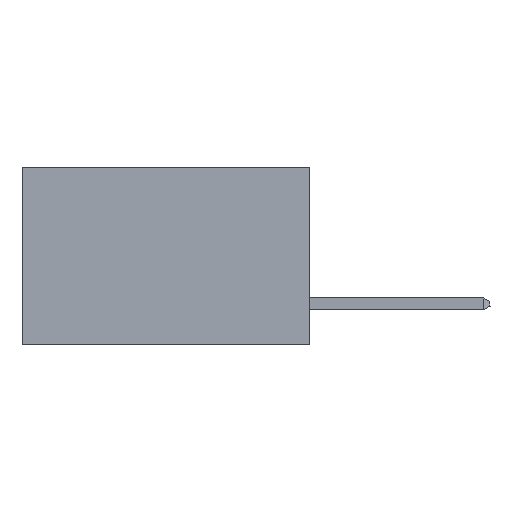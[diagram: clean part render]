
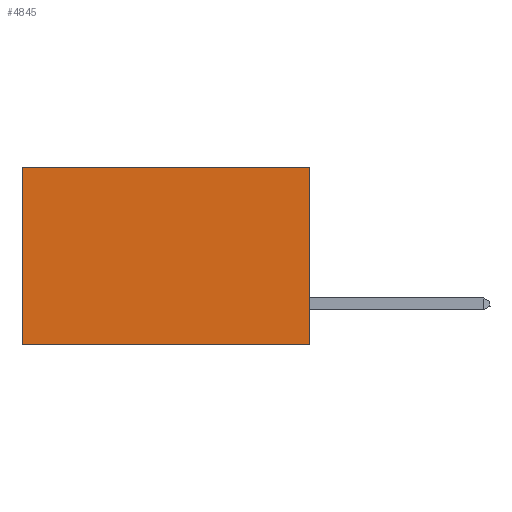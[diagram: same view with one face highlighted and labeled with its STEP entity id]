
A CAD part, left-side view. The second image highlights one B-rep face of the part: STEP entity #4845.
In plain terms, the highlighted planar face has unit normal (-1, 0, 0).
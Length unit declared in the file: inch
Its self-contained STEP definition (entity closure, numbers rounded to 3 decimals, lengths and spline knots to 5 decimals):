
#11 = DIRECTION ( 'NONE',  ( 1., 0., 0. ) ) ;
#539 = DIRECTION ( 'NONE',  ( 0., 0., -1. ) ) ;
#1568 = EDGE_CURVE ( 'NONE', #9355, #11065, #21400, .T. ) ;
#2345 = VECTOR ( 'NONE', #539, 39.37008 ) ;
#4845 = ADVANCED_FACE ( 'NONE', ( #22166 ), #24320, .F. ) ;
#6157 = CARTESIAN_POINT ( 'NONE',  ( 0.2875, 0., 0. ) ) ;
#6753 = VECTOR ( 'NONE', #21107, 39.37008 ) ;
#7283 = CARTESIAN_POINT ( 'NONE',  ( 0.2875, 0.6, -0.37 ) ) ;
#7383 = DIRECTION ( 'NONE',  ( 0., 1., 0. ) ) ;
#7842 = LINE ( 'NONE', #13185, #17094 ) ;
#9315 = CARTESIAN_POINT ( 'NONE',  ( 0.2875, 0.6, 0. ) ) ;
#9355 = VERTEX_POINT ( 'NONE', #9315 ) ;
#10153 = ORIENTED_EDGE ( 'NONE', *, *, #1568, .T. ) ;
#11065 = VERTEX_POINT ( 'NONE', #7283 ) ;
#11925 = CARTESIAN_POINT ( 'NONE',  ( 0.2875, 0., -0.37 ) ) ;
#12388 = VERTEX_POINT ( 'NONE', #22197 ) ;
#13166 = LINE ( 'NONE', #17033, #2345 ) ;
#13185 = CARTESIAN_POINT ( 'NONE',  ( 0.2875, 0., 0. ) ) ;
#14162 = DIRECTION ( 'NONE',  ( 0., 0., -1. ) ) ;
#14805 = EDGE_CURVE ( 'NONE', #12388, #19370, #13166, .T. ) ;
#14972 = CARTESIAN_POINT ( 'NONE',  ( 0.2875, 0.6, 0. ) ) ;
#15254 = EDGE_CURVE ( 'NONE', #19370, #11065, #22708, .T. ) ;
#15750 = ORIENTED_EDGE ( 'NONE', *, *, #19191, .T. ) ;
#17033 = CARTESIAN_POINT ( 'NONE',  ( 0.2875, 0., 0. ) ) ;
#17094 = VECTOR ( 'NONE', #7383, 39.37008 ) ;
#18484 = EDGE_LOOP ( 'NONE', ( #10153, #21695, #21999, #15750 ) ) ;
#19191 = EDGE_CURVE ( 'NONE', #12388, #9355, #7842, .T. ) ;
#19370 = VERTEX_POINT ( 'NONE', #11925 ) ;
#21107 = DIRECTION ( 'NONE',  ( 0., 0., -1. ) ) ;
#21400 = LINE ( 'NONE', #14972, #6753 ) ;
#21695 = ORIENTED_EDGE ( 'NONE', *, *, #15254, .F. ) ;
#21999 = ORIENTED_EDGE ( 'NONE', *, *, #14805, .F. ) ;
#22166 = FACE_OUTER_BOUND ( 'NONE', #18484, .T. ) ;
#22197 = CARTESIAN_POINT ( 'NONE',  ( 0.2875, 0., 0. ) ) ;
#22432 = CARTESIAN_POINT ( 'NONE',  ( 0.2875, 0., -0.37 ) ) ;
#22619 = DIRECTION ( 'NONE',  ( 0., 1., 0. ) ) ;
#22708 = LINE ( 'NONE', #22432, #23654 ) ;
#23654 = VECTOR ( 'NONE', #22619, 39.37008 ) ;
#24320 = PLANE ( 'NONE',  #25611 ) ;
#25611 = AXIS2_PLACEMENT_3D ( 'NONE', #6157, #11, #14162 ) ;
